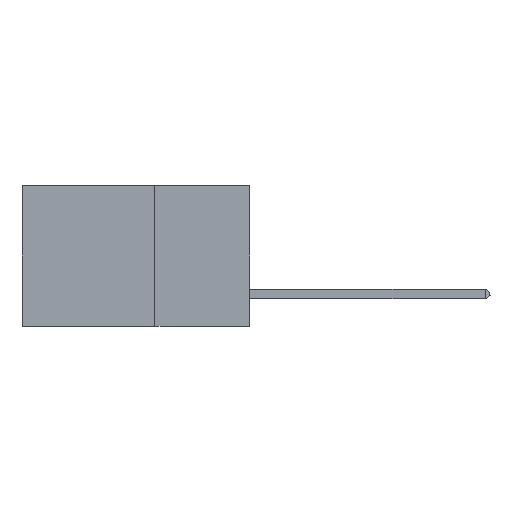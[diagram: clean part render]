
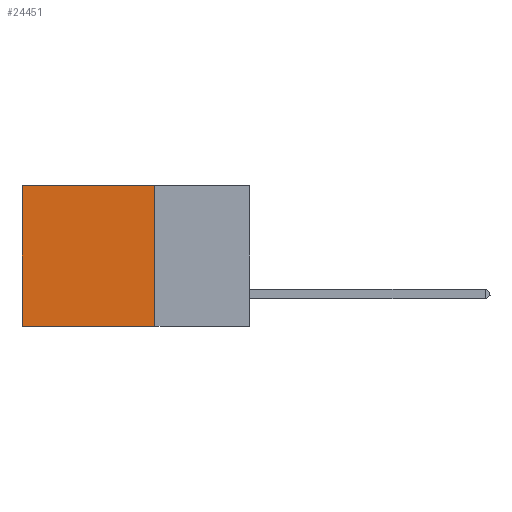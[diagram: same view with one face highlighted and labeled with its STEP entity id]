
A CAD part, left-side view. The second image highlights one B-rep face of the part: STEP entity #24451.
In plain terms, the highlighted planar face has unit normal (-1, 0, 0).
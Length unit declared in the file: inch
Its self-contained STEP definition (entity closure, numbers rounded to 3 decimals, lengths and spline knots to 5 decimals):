
#1982 = CARTESIAN_POINT ( 'NONE',  ( 0.2875, 0.25, -0.37 ) ) ;
#3114 = VERTEX_POINT ( 'NONE', #43888 ) ;
#3796 = CARTESIAN_POINT ( 'NONE',  ( 0.2875, 0.25, 0. ) ) ;
#4672 = CARTESIAN_POINT ( 'NONE',  ( 0.2875, 0.6, 0. ) ) ;
#5256 = PLANE ( 'NONE',  #20118 ) ;
#6414 = VERTEX_POINT ( 'NONE', #1982 ) ;
#8491 = DIRECTION ( 'NONE',  ( 0., 0., -1. ) ) ;
#9032 = CARTESIAN_POINT ( 'NONE',  ( 0.2875, 0.6, 0. ) ) ;
#9302 = LINE ( 'NONE', #35916, #16766 ) ;
#10091 = VERTEX_POINT ( 'NONE', #9032 ) ;
#16766 = VECTOR ( 'NONE', #23807, 39.37008 ) ;
#19122 = EDGE_CURVE ( 'NONE', #6414, #35052, #20885, .T. ) ;
#20118 = AXIS2_PLACEMENT_3D ( 'NONE', #44784, #33350, #45290 ) ;
#20885 = LINE ( 'NONE', #33162, #28305 ) ;
#21217 = EDGE_LOOP ( 'NONE', ( #34585, #32757, #23912, #28666 ) ) ;
#23210 = CARTESIAN_POINT ( 'NONE',  ( 0.2875, 0.6, -0.37 ) ) ;
#23807 = DIRECTION ( 'NONE',  ( 0., 0., -1. ) ) ;
#23912 = ORIENTED_EDGE ( 'NONE', *, *, #39997, .F. ) ;
#23996 = VECTOR ( 'NONE', #27066, 39.37008 ) ;
#24451 = ADVANCED_FACE ( 'NONE', ( #50407 ), #5256, .F. ) ;
#27066 = DIRECTION ( 'NONE',  ( 0., 1., 0. ) ) ;
#28305 = VECTOR ( 'NONE', #48426, 39.37008 ) ;
#28666 = ORIENTED_EDGE ( 'NONE', *, *, #50594, .T. ) ;
#30153 = VECTOR ( 'NONE', #8491, 39.37008 ) ;
#32757 = ORIENTED_EDGE ( 'NONE', *, *, #19122, .F. ) ;
#33162 = CARTESIAN_POINT ( 'NONE',  ( 0.2875, 0.25, -0.37 ) ) ;
#33350 = DIRECTION ( 'NONE',  ( 1., 0., 0. ) ) ;
#34585 = ORIENTED_EDGE ( 'NONE', *, *, #44559, .T. ) ;
#35052 = VERTEX_POINT ( 'NONE', #23210 ) ;
#35916 = CARTESIAN_POINT ( 'NONE',  ( 0.2875, 0.25, 0. ) ) ;
#39997 = EDGE_CURVE ( 'NONE', #3114, #6414, #9302, .T. ) ;
#41931 = LINE ( 'NONE', #4672, #30153 ) ;
#43888 = CARTESIAN_POINT ( 'NONE',  ( 0.2875, 0.25, 0. ) ) ;
#44559 = EDGE_CURVE ( 'NONE', #10091, #35052, #41931, .T. ) ;
#44784 = CARTESIAN_POINT ( 'NONE',  ( 0.2875, 0.25, 0. ) ) ;
#45070 = LINE ( 'NONE', #3796, #23996 ) ;
#45290 = DIRECTION ( 'NONE',  ( 0., 0., -1. ) ) ;
#48426 = DIRECTION ( 'NONE',  ( 0., 1., 0. ) ) ;
#50407 = FACE_OUTER_BOUND ( 'NONE', #21217, .T. ) ;
#50594 = EDGE_CURVE ( 'NONE', #3114, #10091, #45070, .T. ) ;
